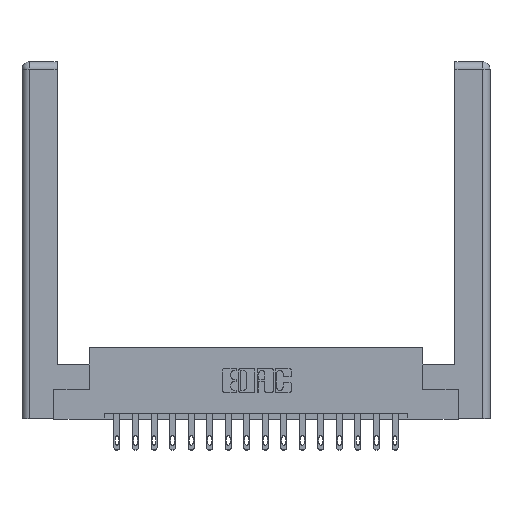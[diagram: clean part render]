
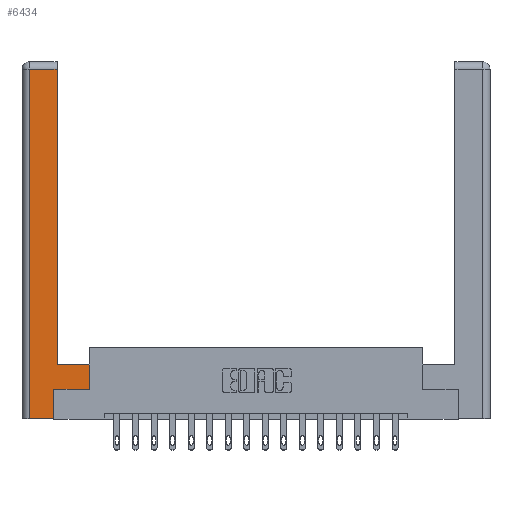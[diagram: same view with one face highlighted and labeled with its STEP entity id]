
A CAD part, top view. The second image highlights one B-rep face of the part: STEP entity #6434.
In plain terms, the highlighted planar face has unit normal (0, 0, 1).
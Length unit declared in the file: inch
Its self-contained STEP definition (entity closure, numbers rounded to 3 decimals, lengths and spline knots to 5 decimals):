
#159 = VERTEX_POINT ( 'NONE', #3124 ) ;
#264 = VERTEX_POINT ( 'NONE', #13047 ) ;
#325 = VECTOR ( 'NONE', #9463, 39.37008 ) ;
#991 = LINE ( 'NONE', #12745, #14469 ) ;
#1074 = CARTESIAN_POINT ( 'NONE',  ( 0.565, 0.45, 0. ) ) ;
#1776 = EDGE_CURVE ( 'NONE', #5130, #12458, #991, .T. ) ;
#2006 = EDGE_CURVE ( 'NONE', #159, #8940, #11384, .T. ) ;
#2063 = DIRECTION ( 'NONE',  ( -1., 0., 0. ) ) ;
#2341 = CARTESIAN_POINT ( 'NONE',  ( 0.295, 3., 0. ) ) ;
#2416 = PLANE ( 'NONE',  #9654 ) ;
#2840 = DIRECTION ( 'NONE',  ( -1., 0., 0. ) ) ;
#3124 = CARTESIAN_POINT ( 'NONE',  ( 0.0615, 2.94, 0. ) ) ;
#3285 = VECTOR ( 'NONE', #8660, 39.37008 ) ;
#3346 = CARTESIAN_POINT ( 'NONE',  ( 0.265, 0., 0. ) ) ;
#3459 = LINE ( 'NONE', #12024, #8780 ) ;
#3850 = VERTEX_POINT ( 'NONE', #3346 ) ;
#4023 = VERTEX_POINT ( 'NONE', #12727 ) ;
#4439 = CARTESIAN_POINT ( 'NONE',  ( 0.0615, 2.94, 0. ) ) ;
#5130 = VERTEX_POINT ( 'NONE', #7749 ) ;
#5534 = CARTESIAN_POINT ( 'NONE',  ( 0., 0., 0. ) ) ;
#6434 = ADVANCED_FACE ( 'NONE', ( #6807 ), #2416, .F. ) ;
#6578 = CARTESIAN_POINT ( 'NONE',  ( 0.0615, 0., 0. ) ) ;
#6700 = EDGE_CURVE ( 'NONE', #3850, #5130, #3459, .T. ) ;
#6807 = FACE_OUTER_BOUND ( 'NONE', #6913, .T. ) ;
#6913 = EDGE_LOOP ( 'NONE', ( #8241, #14749, #7151, #8258, #8532, #9037, #15065, #13602 ) ) ;
#7070 = DIRECTION ( 'NONE',  ( 1., 0., 0. ) ) ;
#7151 = ORIENTED_EDGE ( 'NONE', *, *, #2006, .T. ) ;
#7517 = LINE ( 'NONE', #4439, #3285 ) ;
#7749 = CARTESIAN_POINT ( 'NONE',  ( 0.265, 0.245, 0. ) ) ;
#7960 = EDGE_CURVE ( 'NONE', #12458, #8835, #12063, .T. ) ;
#8170 = CARTESIAN_POINT ( 'NONE',  ( 0.565, 0.245, 0. ) ) ;
#8241 = ORIENTED_EDGE ( 'NONE', *, *, #14648, .T. ) ;
#8258 = ORIENTED_EDGE ( 'NONE', *, *, #14389, .T. ) ;
#8532 = ORIENTED_EDGE ( 'NONE', *, *, #6700, .T. ) ;
#8660 = DIRECTION ( 'NONE',  ( -1., 0., 0. ) ) ;
#8780 = VECTOR ( 'NONE', #9034, 39.37008 ) ;
#8835 = VERTEX_POINT ( 'NONE', #17573 ) ;
#8940 = VERTEX_POINT ( 'NONE', #6578 ) ;
#9034 = DIRECTION ( 'NONE',  ( 0., 1., 0. ) ) ;
#9037 = ORIENTED_EDGE ( 'NONE', *, *, #1776, .T. ) ;
#9168 = CARTESIAN_POINT ( 'NONE',  ( 0.295, 0.45, 0. ) ) ;
#9463 = DIRECTION ( 'NONE',  ( 0., 1., 0. ) ) ;
#9654 = AXIS2_PLACEMENT_3D ( 'NONE', #5534, #15634, #2840 ) ;
#9738 = EDGE_CURVE ( 'NONE', #8835, #4023, #14748, .T. ) ;
#10311 = VECTOR ( 'NONE', #17608, 39.37008 ) ;
#11384 = LINE ( 'NONE', #17592, #11832 ) ;
#11832 = VECTOR ( 'NONE', #11896, 39.37008 ) ;
#11896 = DIRECTION ( 'NONE',  ( 0., -1., 0. ) ) ;
#12024 = CARTESIAN_POINT ( 'NONE',  ( 0.265, 0.245, 0. ) ) ;
#12063 = LINE ( 'NONE', #1074, #16281 ) ;
#12458 = VERTEX_POINT ( 'NONE', #8170 ) ;
#12727 = CARTESIAN_POINT ( 'NONE',  ( 0.295, 0.45, 0. ) ) ;
#12745 = CARTESIAN_POINT ( 'NONE',  ( 0.565, 0.245, 0. ) ) ;
#13047 = CARTESIAN_POINT ( 'NONE',  ( 0.295, 2.94, 0. ) ) ;
#13572 = DIRECTION ( 'NONE',  ( 0., 1., 0. ) ) ;
#13602 = ORIENTED_EDGE ( 'NONE', *, *, #9738, .T. ) ;
#14389 = EDGE_CURVE ( 'NONE', #8940, #3850, #16980, .T. ) ;
#14469 = VECTOR ( 'NONE', #7070, 39.37008 ) ;
#14648 = EDGE_CURVE ( 'NONE', #4023, #264, #18289, .T. ) ;
#14748 = LINE ( 'NONE', #9168, #16546 ) ;
#14749 = ORIENTED_EDGE ( 'NONE', *, *, #16045, .T. ) ;
#15065 = ORIENTED_EDGE ( 'NONE', *, *, #7960, .T. ) ;
#15634 = DIRECTION ( 'NONE',  ( 0., 0., -1. ) ) ;
#16045 = EDGE_CURVE ( 'NONE', #264, #159, #7517, .T. ) ;
#16066 = CARTESIAN_POINT ( 'NONE',  ( 0.265, 0., 0. ) ) ;
#16281 = VECTOR ( 'NONE', #13572, 39.37008 ) ;
#16546 = VECTOR ( 'NONE', #2063, 39.37008 ) ;
#16980 = LINE ( 'NONE', #16066, #10311 ) ;
#17573 = CARTESIAN_POINT ( 'NONE',  ( 0.565, 0.45, 0. ) ) ;
#17592 = CARTESIAN_POINT ( 'NONE',  ( 0.0615, 0., 0. ) ) ;
#17608 = DIRECTION ( 'NONE',  ( 1., 0., 0. ) ) ;
#18289 = LINE ( 'NONE', #2341, #325 ) ;
